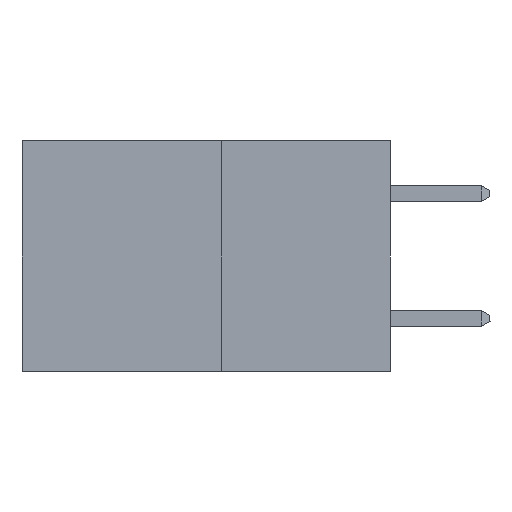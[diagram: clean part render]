
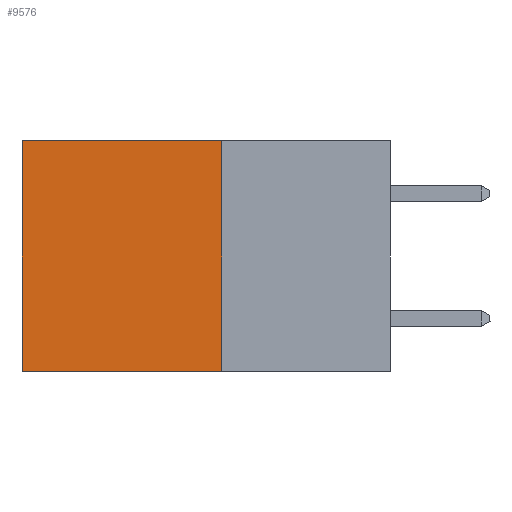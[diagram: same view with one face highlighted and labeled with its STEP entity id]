
A CAD part, left-side view. The second image highlights one B-rep face of the part: STEP entity #9576.
In plain terms, the highlighted planar face has unit normal (-1, 0, 0).
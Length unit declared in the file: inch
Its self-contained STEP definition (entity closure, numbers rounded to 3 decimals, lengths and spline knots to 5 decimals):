
#903 = DIRECTION ( 'NONE',  ( 0., 1., 0. ) ) ;
#1383 = CARTESIAN_POINT ( 'NONE',  ( 0.277, 0.27, 0. ) ) ;
#2138 = CARTESIAN_POINT ( 'NONE',  ( 0.277, 0.27, -0.37 ) ) ;
#2230 = EDGE_CURVE ( 'NONE', #13138, #21258, #6193, .T. ) ;
#5526 = ORIENTED_EDGE ( 'NONE', *, *, #2230, .T. ) ;
#5634 = LINE ( 'NONE', #2138, #14959 ) ;
#5786 = CARTESIAN_POINT ( 'NONE',  ( 0.277, 0.27, -0.37 ) ) ;
#6193 = LINE ( 'NONE', #6208, #19136 ) ;
#6208 = CARTESIAN_POINT ( 'NONE',  ( 0.277, 0.59, -0.37 ) ) ;
#6660 = DIRECTION ( 'NONE',  ( 1., 0., 0. ) ) ;
#6691 = AXIS2_PLACEMENT_3D ( 'NONE', #17195, #6660, #18963 ) ;
#7356 = CARTESIAN_POINT ( 'NONE',  ( 0.277, 0.59, 0. ) ) ;
#7734 = ORIENTED_EDGE ( 'NONE', *, *, #16720, .F. ) ;
#8111 = FACE_OUTER_BOUND ( 'NONE', #11630, .T. ) ;
#8917 = ORIENTED_EDGE ( 'NONE', *, *, #9236, .T. ) ;
#9236 = EDGE_CURVE ( 'NONE', #22476, #13138, #15253, .T. ) ;
#9362 = CARTESIAN_POINT ( 'NONE',  ( 0.277, 0.27, 0. ) ) ;
#9489 = CARTESIAN_POINT ( 'NONE',  ( 0.277, 0.59, -0.37 ) ) ;
#9576 = ADVANCED_FACE ( 'NONE', ( #8111 ), #22452, .F. ) ;
#10547 = VECTOR ( 'NONE', #903, 39.37008 ) ;
#10859 = CARTESIAN_POINT ( 'NONE',  ( 0.277, 0.27, -0.37 ) ) ;
#11630 = EDGE_LOOP ( 'NONE', ( #5526, #17864, #7734, #8917 ) ) ;
#13138 = VERTEX_POINT ( 'NONE', #7356 ) ;
#13200 = VERTEX_POINT ( 'NONE', #5786 ) ;
#13723 = VECTOR ( 'NONE', #16283, 39.37008 ) ;
#14441 = DIRECTION ( 'NONE',  ( 0., 1., 0. ) ) ;
#14959 = VECTOR ( 'NONE', #14441, 39.37008 ) ;
#15253 = LINE ( 'NONE', #1383, #10547 ) ;
#16283 = DIRECTION ( 'NONE',  ( 0., 0., -1. ) ) ;
#16713 = DIRECTION ( 'NONE',  ( 0., 0., -1. ) ) ;
#16720 = EDGE_CURVE ( 'NONE', #22476, #13200, #18474, .T. ) ;
#17195 = CARTESIAN_POINT ( 'NONE',  ( 0.277, 0.27, -0.37 ) ) ;
#17864 = ORIENTED_EDGE ( 'NONE', *, *, #19681, .F. ) ;
#18474 = LINE ( 'NONE', #10859, #13723 ) ;
#18963 = DIRECTION ( 'NONE',  ( 0., 0., -1. ) ) ;
#19136 = VECTOR ( 'NONE', #16713, 39.37008 ) ;
#19681 = EDGE_CURVE ( 'NONE', #13200, #21258, #5634, .T. ) ;
#21258 = VERTEX_POINT ( 'NONE', #9489 ) ;
#22452 = PLANE ( 'NONE',  #6691 ) ;
#22476 = VERTEX_POINT ( 'NONE', #9362 ) ;
